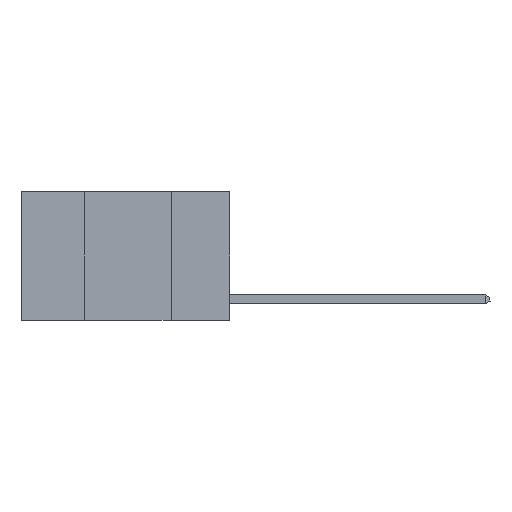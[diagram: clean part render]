
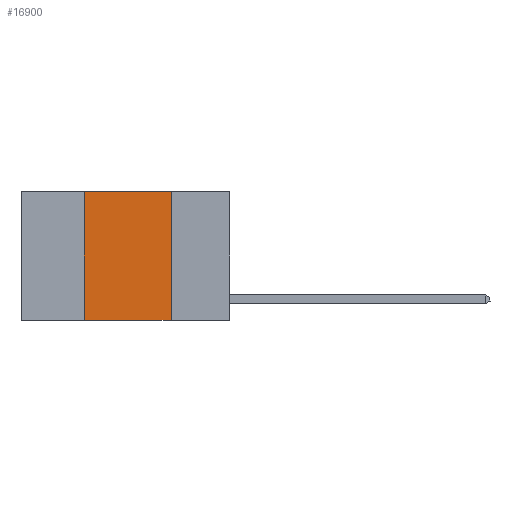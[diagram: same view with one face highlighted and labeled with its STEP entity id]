
A CAD part, left-side view. The second image highlights one B-rep face of the part: STEP entity #16900.
In plain terms, the highlighted planar face has unit normal (-1, 0, 0).
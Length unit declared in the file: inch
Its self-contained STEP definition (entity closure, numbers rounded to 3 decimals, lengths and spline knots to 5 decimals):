
#701 = EDGE_CURVE ( 'NONE', #12969, #5662, #16456, .T. ) ;
#1040 = CARTESIAN_POINT ( 'NONE',  ( 0., 0.6, -0.37 ) ) ;
#2195 = ORIENTED_EDGE ( 'NONE', *, *, #3012, .F. ) ;
#2515 = DIRECTION ( 'NONE',  ( 1., 0., 0. ) ) ;
#3012 = EDGE_CURVE ( 'NONE', #4415, #8536, #15632, .T. ) ;
#3843 = AXIS2_PLACEMENT_3D ( 'NONE', #23124, #2515, #17091 ) ;
#4415 = VERTEX_POINT ( 'NONE', #12552 ) ;
#5662 = VERTEX_POINT ( 'NONE', #8381 ) ;
#5882 = EDGE_LOOP ( 'NONE', ( #11300, #2195, #15213, #25422 ) ) ;
#6404 = EDGE_CURVE ( 'NONE', #8536, #5662, #20892, .T. ) ;
#8381 = CARTESIAN_POINT ( 'NONE',  ( 0., 0.17, -0.37 ) ) ;
#8536 = VERTEX_POINT ( 'NONE', #23597 ) ;
#9477 = CARTESIAN_POINT ( 'NONE',  ( 0., 0.6, 0. ) ) ;
#10117 = DIRECTION ( 'NONE',  ( 0., -1., 0. ) ) ;
#10150 = VECTOR ( 'NONE', #19785, 39.37008 ) ;
#11300 = ORIENTED_EDGE ( 'NONE', *, *, #6404, .F. ) ;
#12277 = CARTESIAN_POINT ( 'NONE',  ( 0., 0.42, 0. ) ) ;
#12552 = CARTESIAN_POINT ( 'NONE',  ( 0., 0.42, 0. ) ) ;
#12969 = VERTEX_POINT ( 'NONE', #25853 ) ;
#13004 = DIRECTION ( 'NONE',  ( 0., 0., -1. ) ) ;
#14418 = LINE ( 'NONE', #12277, #26106 ) ;
#15149 = VECTOR ( 'NONE', #10117, 39.37008 ) ;
#15213 = ORIENTED_EDGE ( 'NONE', *, *, #20471, .F. ) ;
#15445 = VECTOR ( 'NONE', #13004, 39.37008 ) ;
#15632 = LINE ( 'NONE', #9477, #10150 ) ;
#16456 = LINE ( 'NONE', #1040, #15149 ) ;
#16769 = FACE_OUTER_BOUND ( 'NONE', #5882, .T. ) ;
#16900 = ADVANCED_FACE ( 'NONE', ( #16769 ), #16998, .F. ) ;
#16998 = PLANE ( 'NONE',  #3843 ) ;
#17091 = DIRECTION ( 'NONE',  ( 0., 0., -1. ) ) ;
#18515 = DIRECTION ( 'NONE',  ( 0., 0., 1. ) ) ;
#19785 = DIRECTION ( 'NONE',  ( 0., -1., 0. ) ) ;
#20471 = EDGE_CURVE ( 'NONE', #12969, #4415, #14418, .T. ) ;
#20892 = LINE ( 'NONE', #21121, #15445 ) ;
#21121 = CARTESIAN_POINT ( 'NONE',  ( 0., 0.17, 0. ) ) ;
#23124 = CARTESIAN_POINT ( 'NONE',  ( 0., 0.6, 0. ) ) ;
#23597 = CARTESIAN_POINT ( 'NONE',  ( 0., 0.17, 0. ) ) ;
#25422 = ORIENTED_EDGE ( 'NONE', *, *, #701, .T. ) ;
#25853 = CARTESIAN_POINT ( 'NONE',  ( 0., 0.42, -0.37 ) ) ;
#26106 = VECTOR ( 'NONE', #18515, 39.37008 ) ;
